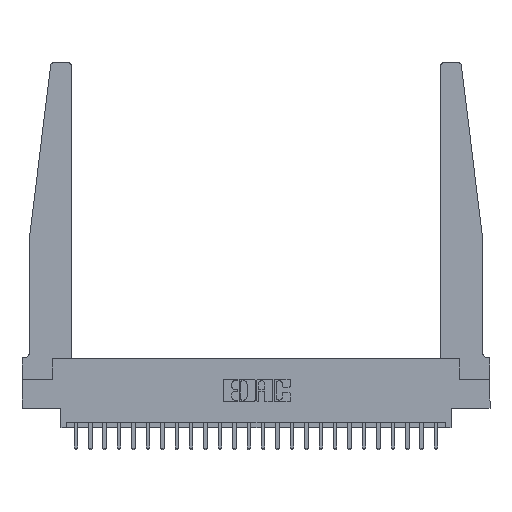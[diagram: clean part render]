
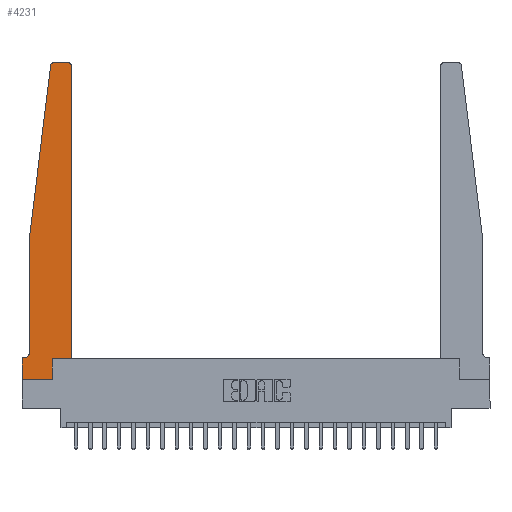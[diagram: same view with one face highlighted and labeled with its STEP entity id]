
A CAD part, top view. The second image highlights one B-rep face of the part: STEP entity #4231.
In plain terms, the highlighted planar face has unit normal (0, 0, 1).
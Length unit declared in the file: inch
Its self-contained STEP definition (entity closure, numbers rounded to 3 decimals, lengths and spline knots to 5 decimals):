
#228 = DIRECTION ( 'NONE',  ( -1., 0., 0. ) ) ;
#515 = VERTEX_POINT ( 'NONE', #12994 ) ;
#544 = CARTESIAN_POINT ( 'NONE',  ( 0.065, 0.1875, 0.37 ) ) ;
#577 = LINE ( 'NONE', #19112, #13577 ) ;
#868 = CARTESIAN_POINT ( 'NONE',  ( 0., 0., 0.37 ) ) ;
#881 = ORIENTED_EDGE ( 'NONE', *, *, #16390, .T. ) ;
#1109 = CARTESIAN_POINT ( 'NONE',  ( 0.065, 0.2375, 0.37 ) ) ;
#1478 = VERTEX_POINT ( 'NONE', #22023 ) ;
#2012 = ORIENTED_EDGE ( 'NONE', *, *, #21069, .T. ) ;
#2812 = DIRECTION ( 'NONE',  ( 0., -1., 0. ) ) ;
#2815 = DIRECTION ( 'NONE',  ( 0., 0., 1. ) ) ;
#2852 = VERTEX_POINT ( 'NONE', #3694 ) ;
#3041 = ORIENTED_EDGE ( 'NONE', *, *, #10307, .T. ) ;
#3056 = VECTOR ( 'NONE', #3212, 39.37008 ) ;
#3066 = CARTESIAN_POINT ( 'NONE',  ( 0.065, 1.25, 0.37 ) ) ;
#3119 = CARTESIAN_POINT ( 'NONE',  ( 0.015, 0.2375, 0.37 ) ) ;
#3212 = DIRECTION ( 'NONE',  ( 1., 0., 0. ) ) ;
#3588 = DIRECTION ( 'NONE',  ( 0., 0., 1. ) ) ;
#3694 = CARTESIAN_POINT ( 'NONE',  ( 0., 0.1875, 0.37 ) ) ;
#3983 = ORIENTED_EDGE ( 'NONE', *, *, #8248, .T. ) ;
#4231 = ADVANCED_FACE ( 'NONE', ( #16368 ), #9620, .T. ) ;
#4322 = VECTOR ( 'NONE', #8232, 39.37008 ) ;
#4446 = DIRECTION ( 'NONE',  ( -1., 0., 0. ) ) ;
#4575 = LINE ( 'NONE', #544, #18997 ) ;
#4610 = ORIENTED_EDGE ( 'NONE', *, *, #23395, .T. ) ;
#5047 = DIRECTION ( 'NONE',  ( -1., 0., 0. ) ) ;
#5105 = DIRECTION ( 'NONE',  ( 0., -1., 0. ) ) ;
#6254 = VECTOR ( 'NONE', #5105, 39.37008 ) ;
#6371 = VECTOR ( 'NONE', #2812, 39.37008 ) ;
#6561 = CARTESIAN_POINT ( 'NONE',  ( 0.2605, 0.18, 0.37 ) ) ;
#6830 = VERTEX_POINT ( 'NONE', #9638 ) ;
#7044 = CIRCLE ( 'NONE', #19218, 0.03 ) ;
#7101 = ORIENTED_EDGE ( 'NONE', *, *, #17478, .T. ) ;
#7734 = AXIS2_PLACEMENT_3D ( 'NONE', #24141, #22475, #11522 ) ;
#7986 = CARTESIAN_POINT ( 'NONE',  ( 0.395, 2.75, 0.37 ) ) ;
#8111 = ORIENTED_EDGE ( 'NONE', *, *, #9396, .T. ) ;
#8165 = VERTEX_POINT ( 'NONE', #7986 ) ;
#8232 = DIRECTION ( 'NONE',  ( 0., 1., 0. ) ) ;
#8248 = EDGE_CURVE ( 'NONE', #21093, #8355, #14440, .T. ) ;
#8355 = VERTEX_POINT ( 'NONE', #8552 ) ;
#8357 = EDGE_CURVE ( 'NONE', #1478, #16165, #7044, .T. ) ;
#8480 = DIRECTION ( 'NONE',  ( 0., 1., 0. ) ) ;
#8552 = CARTESIAN_POINT ( 'NONE',  ( 0.425, 2.72, 0.37 ) ) ;
#8776 = LINE ( 'NONE', #18354, #3056 ) ;
#8791 = VERTEX_POINT ( 'NONE', #1109 ) ;
#8954 = DIRECTION ( 'NONE',  ( -0.122, -0.992, 0. ) ) ;
#9396 = EDGE_CURVE ( 'NONE', #6830, #21093, #8776, .T. ) ;
#9559 = LINE ( 'NONE', #3066, #19999 ) ;
#9620 = PLANE ( 'NONE',  #7734 ) ;
#9638 = CARTESIAN_POINT ( 'NONE',  ( 0.2605, 0.18, 0.37 ) ) ;
#10285 = CARTESIAN_POINT ( 'NONE',  ( 0.2605, 0., 0.37 ) ) ;
#10307 = EDGE_CURVE ( 'NONE', #18264, #2852, #4575, .T. ) ;
#10597 = CARTESIAN_POINT ( 'NONE',  ( 0.24675, 2.72367, 0.37 ) ) ;
#11522 = DIRECTION ( 'NONE',  ( 1., 0., 0. ) ) ;
#12667 = CIRCLE ( 'NONE', #16476, 0.05 ) ;
#12994 = CARTESIAN_POINT ( 'NONE',  ( 0., 0., 0.37 ) ) ;
#13399 = EDGE_LOOP ( 'NONE', ( #15300, #20536, #4610, #7101, #18929, #3041, #2012, #20052, #22731, #8111, #3983, #881 ) ) ;
#13577 = VECTOR ( 'NONE', #228, 39.37008 ) ;
#13726 = LINE ( 'NONE', #21814, #22824 ) ;
#14111 = CARTESIAN_POINT ( 'NONE',  ( 0.065, 1.25, 0.37 ) ) ;
#14243 = CARTESIAN_POINT ( 'NONE',  ( 0.27653, 2.72, 0.37 ) ) ;
#14314 = CIRCLE ( 'NONE', #15326, 0.03 ) ;
#14440 = LINE ( 'NONE', #17573, #4322 ) ;
#15004 = CARTESIAN_POINT ( 'NONE',  ( 0.395, 2.72, 0.37 ) ) ;
#15300 = ORIENTED_EDGE ( 'NONE', *, *, #22046, .T. ) ;
#15326 = AXIS2_PLACEMENT_3D ( 'NONE', #15004, #3588, #16870 ) ;
#16122 = CARTESIAN_POINT ( 'NONE',  ( 0.425, 0.18, 0.37 ) ) ;
#16127 = DIRECTION ( 'NONE',  ( 1., 0., 0. ) ) ;
#16165 = VERTEX_POINT ( 'NONE', #10597 ) ;
#16306 = LINE ( 'NONE', #23550, #6254 ) ;
#16368 = FACE_OUTER_BOUND ( 'NONE', #13399, .T. ) ;
#16390 = EDGE_CURVE ( 'NONE', #8355, #8165, #14314, .T. ) ;
#16404 = DIRECTION ( 'NONE',  ( 0., 0., -1. ) ) ;
#16418 = LINE ( 'NONE', #868, #6371 ) ;
#16476 = AXIS2_PLACEMENT_3D ( 'NONE', #3119, #16404, #5047 ) ;
#16870 = DIRECTION ( 'NONE',  ( 1., 0., 0. ) ) ;
#17290 = VERTEX_POINT ( 'NONE', #14111 ) ;
#17478 = EDGE_CURVE ( 'NONE', #17290, #8791, #16306, .T. ) ;
#17573 = CARTESIAN_POINT ( 'NONE',  ( 0.425, 0.18, 0.37 ) ) ;
#18264 = VERTEX_POINT ( 'NONE', #22251 ) ;
#18354 = CARTESIAN_POINT ( 'NONE',  ( 0.425, 0.18, 0.37 ) ) ;
#18572 = VERTEX_POINT ( 'NONE', #10285 ) ;
#18929 = ORIENTED_EDGE ( 'NONE', *, *, #20047, .T. ) ;
#18997 = VECTOR ( 'NONE', #4446, 39.37008 ) ;
#19112 = CARTESIAN_POINT ( 'NONE',  ( 0.25, 2.75, 0.37 ) ) ;
#19218 = AXIS2_PLACEMENT_3D ( 'NONE', #14243, #2815, #16127 ) ;
#19999 = VECTOR ( 'NONE', #8954, 39.37008 ) ;
#20047 = EDGE_CURVE ( 'NONE', #8791, #18264, #12667, .T. ) ;
#20052 = ORIENTED_EDGE ( 'NONE', *, *, #22353, .T. ) ;
#20536 = ORIENTED_EDGE ( 'NONE', *, *, #8357, .T. ) ;
#20597 = EDGE_CURVE ( 'NONE', #18572, #6830, #21800, .T. ) ;
#21069 = EDGE_CURVE ( 'NONE', #2852, #515, #16418, .T. ) ;
#21093 = VERTEX_POINT ( 'NONE', #16122 ) ;
#21247 = VECTOR ( 'NONE', #8480, 39.37008 ) ;
#21800 = LINE ( 'NONE', #6561, #21247 ) ;
#21814 = CARTESIAN_POINT ( 'NONE',  ( 0., 0., 0.37 ) ) ;
#22023 = CARTESIAN_POINT ( 'NONE',  ( 0.27653, 2.75, 0.37 ) ) ;
#22046 = EDGE_CURVE ( 'NONE', #8165, #1478, #577, .T. ) ;
#22251 = CARTESIAN_POINT ( 'NONE',  ( 0.015, 0.1875, 0.37 ) ) ;
#22353 = EDGE_CURVE ( 'NONE', #515, #18572, #13726, .T. ) ;
#22475 = DIRECTION ( 'NONE',  ( 0., 0., 1. ) ) ;
#22731 = ORIENTED_EDGE ( 'NONE', *, *, #20597, .T. ) ;
#22824 = VECTOR ( 'NONE', #23549, 39.37008 ) ;
#23395 = EDGE_CURVE ( 'NONE', #16165, #17290, #9559, .T. ) ;
#23549 = DIRECTION ( 'NONE',  ( 1., 0., 0. ) ) ;
#23550 = CARTESIAN_POINT ( 'NONE',  ( 0.065, 1.25, 0.37 ) ) ;
#24141 = CARTESIAN_POINT ( 'NONE',  ( 0., 0.1875, 0.37 ) ) ;
